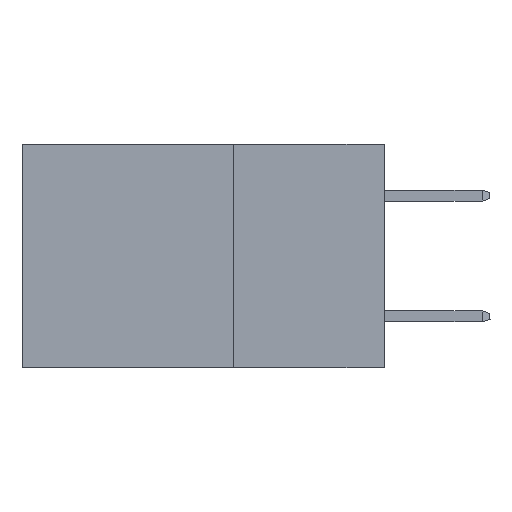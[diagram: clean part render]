
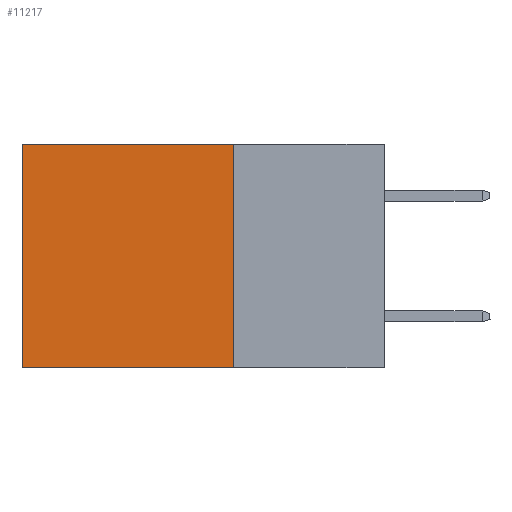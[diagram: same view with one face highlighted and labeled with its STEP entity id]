
A CAD part, left-side view. The second image highlights one B-rep face of the part: STEP entity #11217.
In plain terms, the highlighted planar face has unit normal (-1, 0, 0).
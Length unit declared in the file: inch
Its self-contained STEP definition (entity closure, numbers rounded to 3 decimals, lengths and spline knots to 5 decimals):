
#1067 = VERTEX_POINT ( 'NONE', #8590 ) ;
#1346 = CARTESIAN_POINT ( 'NONE',  ( 0.2615, 0.6, -0.37 ) ) ;
#1568 = EDGE_CURVE ( 'NONE', #18059, #16098, #16049, .T. ) ;
#1590 = ORIENTED_EDGE ( 'NONE', *, *, #17858, .F. ) ;
#2004 = LINE ( 'NONE', #7092, #16601 ) ;
#2046 = LINE ( 'NONE', #11451, #5463 ) ;
#2659 = ORIENTED_EDGE ( 'NONE', *, *, #5283, .T. ) ;
#3931 = CARTESIAN_POINT ( 'NONE',  ( 0.2615, 0.25, -0.37 ) ) ;
#4414 = FACE_OUTER_BOUND ( 'NONE', #8958, .T. ) ;
#4441 = LINE ( 'NONE', #3931, #7821 ) ;
#5089 = CARTESIAN_POINT ( 'NONE',  ( 0.2615, 0.6, -0.37 ) ) ;
#5283 = EDGE_CURVE ( 'NONE', #1067, #18059, #2046, .T. ) ;
#5463 = VECTOR ( 'NONE', #11519, 39.37008 ) ;
#6217 = EDGE_CURVE ( 'NONE', #10499, #16098, #2004, .T. ) ;
#6771 = PLANE ( 'NONE',  #18365 ) ;
#6782 = DIRECTION ( 'NONE',  ( 0., 1., 0. ) ) ;
#7092 = CARTESIAN_POINT ( 'NONE',  ( 0.2615, 0.25, -0.37 ) ) ;
#7262 = CARTESIAN_POINT ( 'NONE',  ( 0.2615, 0.6, 0. ) ) ;
#7821 = VECTOR ( 'NONE', #15310, 39.37008 ) ;
#8198 = DIRECTION ( 'NONE',  ( 1., 0., 0. ) ) ;
#8469 = ORIENTED_EDGE ( 'NONE', *, *, #6217, .F. ) ;
#8590 = CARTESIAN_POINT ( 'NONE',  ( 0.2615, 0.25, 0. ) ) ;
#8958 = EDGE_LOOP ( 'NONE', ( #12861, #8469, #1590, #2659 ) ) ;
#9110 = DIRECTION ( 'NONE',  ( 0., 0., -1. ) ) ;
#10499 = VERTEX_POINT ( 'NONE', #10761 ) ;
#10761 = CARTESIAN_POINT ( 'NONE',  ( 0.2615, 0.25, -0.37 ) ) ;
#11217 = ADVANCED_FACE ( 'NONE', ( #4414 ), #6771, .F. ) ;
#11451 = CARTESIAN_POINT ( 'NONE',  ( 0.2615, 0.25, 0. ) ) ;
#11519 = DIRECTION ( 'NONE',  ( 0., 1., 0. ) ) ;
#12801 = VECTOR ( 'NONE', #9110, 39.37008 ) ;
#12861 = ORIENTED_EDGE ( 'NONE', *, *, #1568, .T. ) ;
#15182 = CARTESIAN_POINT ( 'NONE',  ( 0.2615, 0.25, -0.37 ) ) ;
#15310 = DIRECTION ( 'NONE',  ( 0., 0., -1. ) ) ;
#16049 = LINE ( 'NONE', #5089, #12801 ) ;
#16098 = VERTEX_POINT ( 'NONE', #1346 ) ;
#16601 = VECTOR ( 'NONE', #6782, 39.37008 ) ;
#17858 = EDGE_CURVE ( 'NONE', #1067, #10499, #4441, .T. ) ;
#17900 = DIRECTION ( 'NONE',  ( 0., 0., -1. ) ) ;
#18059 = VERTEX_POINT ( 'NONE', #7262 ) ;
#18365 = AXIS2_PLACEMENT_3D ( 'NONE', #15182, #8198, #17900 ) ;
